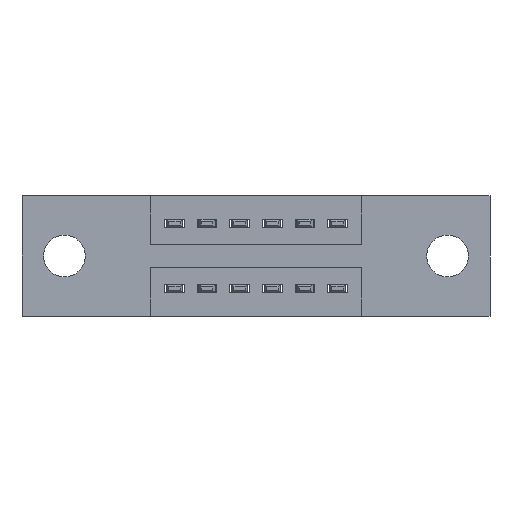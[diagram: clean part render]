
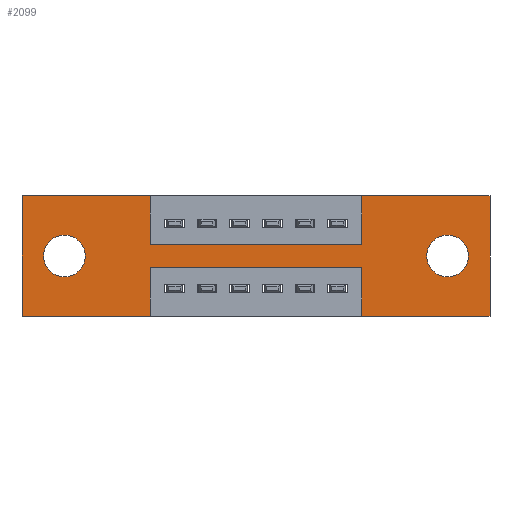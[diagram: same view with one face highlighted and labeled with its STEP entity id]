
A CAD part, front view. The second image highlights one B-rep face of the part: STEP entity #2099.
In plain terms, the highlighted planar face has unit normal (0, -1, 0).
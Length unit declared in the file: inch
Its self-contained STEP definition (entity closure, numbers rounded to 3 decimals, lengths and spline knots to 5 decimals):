
#1 = DIRECTION ( 'NONE',  ( 0., 1., 0. ) ) ;
#26 = CARTESIAN_POINT ( 'NONE',  ( 0., 0., 0. ) ) ;
#52 = EDGE_CURVE ( 'NONE', #2543, #3641, #4441, .T. ) ;
#180 = DIRECTION ( 'NONE',  ( 0., 0., -1. ) ) ;
#314 = VECTOR ( 'NONE', #6771, 39.37008 ) ;
#484 = AXIS2_PLACEMENT_3D ( 'NONE', #5049, #4975, #4965 ) ;
#531 = CARTESIAN_POINT ( 'NONE',  ( 1.305, 0., -0.185 ) ) ;
#575 = DIRECTION ( 'NONE',  ( 0., 0., 1. ) ) ;
#579 = ORIENTED_EDGE ( 'NONE', *, *, #7666, .T. ) ;
#630 = AXIS2_PLACEMENT_3D ( 'NONE', #892, #879, #575 ) ;
#729 = ORIENTED_EDGE ( 'NONE', *, *, #5892, .F. ) ;
#764 = VECTOR ( 'NONE', #1895, 39.37008 ) ;
#770 = LINE ( 'NONE', #5161, #6510 ) ;
#814 = LINE ( 'NONE', #9161, #8529 ) ;
#859 = ORIENTED_EDGE ( 'NONE', *, *, #7295, .F. ) ;
#872 = CARTESIAN_POINT ( 'NONE',  ( 0.3925, 0., -0.37 ) ) ;
#879 = DIRECTION ( 'NONE',  ( 0., 1., 0. ) ) ;
#892 = CARTESIAN_POINT ( 'NONE',  ( 0.13, 0., -0.185 ) ) ;
#940 = VERTEX_POINT ( 'NONE', #3527 ) ;
#981 = VERTEX_POINT ( 'NONE', #2185 ) ;
#990 = ORIENTED_EDGE ( 'NONE', *, *, #2960, .T. ) ;
#1018 = ORIENTED_EDGE ( 'NONE', *, *, #2408, .T. ) ;
#1060 = EDGE_CURVE ( 'NONE', #2987, #3016, #2873, .T. ) ;
#1078 = ORIENTED_EDGE ( 'NONE', *, *, #1060, .F. ) ;
#1226 = ORIENTED_EDGE ( 'NONE', *, *, #8781, .F. ) ;
#1514 = CIRCLE ( 'NONE', #484, 0.064 ) ;
#1549 = ORIENTED_EDGE ( 'NONE', *, *, #4162, .F. ) ;
#1569 = EDGE_LOOP ( 'NONE', ( #990, #1018 ) ) ;
#1657 = ORIENTED_EDGE ( 'NONE', *, *, #9216, .F. ) ;
#1735 = VERTEX_POINT ( 'NONE', #6779 ) ;
#1806 = ORIENTED_EDGE ( 'NONE', *, *, #8166, .F. ) ;
#1809 = DIRECTION ( 'NONE',  ( 0., 0., -1. ) ) ;
#1895 = DIRECTION ( 'NONE',  ( 0., 0., 1. ) ) ;
#1947 = CARTESIAN_POINT ( 'NONE',  ( 1.0425, 0., 0. ) ) ;
#2099 = ADVANCED_FACE ( 'NONE', ( #2370, #7669, #4164 ), #7871, .T. ) ;
#2115 = ORIENTED_EDGE ( 'NONE', *, *, #4120, .F. ) ;
#2185 = CARTESIAN_POINT ( 'NONE',  ( 1.435, 0., -0.37 ) ) ;
#2215 = VERTEX_POINT ( 'NONE', #6495 ) ;
#2240 = CARTESIAN_POINT ( 'NONE',  ( 1.435, 0., 0. ) ) ;
#2258 = ORIENTED_EDGE ( 'NONE', *, *, #8066, .F. ) ;
#2370 = FACE_BOUND ( 'NONE', #1569, .T. ) ;
#2408 = EDGE_CURVE ( 'NONE', #2215, #940, #1514, .T. ) ;
#2412 = ORIENTED_EDGE ( 'NONE', *, *, #52, .F. ) ;
#2415 = CARTESIAN_POINT ( 'NONE',  ( 1.0425, 0., -0.37 ) ) ;
#2441 = EDGE_CURVE ( 'NONE', #3881, #3059, #7356, .T. ) ;
#2543 = VERTEX_POINT ( 'NONE', #3955 ) ;
#2873 = LINE ( 'NONE', #2415, #764 ) ;
#2920 = ORIENTED_EDGE ( 'NONE', *, *, #7743, .F. ) ;
#2931 = CARTESIAN_POINT ( 'NONE',  ( 0., 0., 0. ) ) ;
#2960 = EDGE_CURVE ( 'NONE', #940, #2215, #3087, .T. ) ;
#2987 = VERTEX_POINT ( 'NONE', #7639 ) ;
#3016 = VERTEX_POINT ( 'NONE', #6054 ) ;
#3056 = ORIENTED_EDGE ( 'NONE', *, *, #5454, .T. ) ;
#3059 = VERTEX_POINT ( 'NONE', #4786 ) ;
#3087 = CIRCLE ( 'NONE', #7286, 0.064 ) ;
#3143 = CIRCLE ( 'NONE', #630, 0.064 ) ;
#3177 = ORIENTED_EDGE ( 'NONE', *, *, #2441, .F. ) ;
#3354 = VECTOR ( 'NONE', #7906, 39.37008 ) ;
#3527 = CARTESIAN_POINT ( 'NONE',  ( 1.305, 0., -0.121 ) ) ;
#3598 = CARTESIAN_POINT ( 'NONE',  ( 0.13, 0., -0.185 ) ) ;
#3607 = CARTESIAN_POINT ( 'NONE',  ( 0.3925, 0., -0.15 ) ) ;
#3641 = VERTEX_POINT ( 'NONE', #7553 ) ;
#3727 = EDGE_LOOP ( 'NONE', ( #729, #859, #1078, #1226, #1549, #1657, #1806, #2115, #2258, #2412, #2920, #3177 ) ) ;
#3779 = VERTEX_POINT ( 'NONE', #5271 ) ;
#3881 = VERTEX_POINT ( 'NONE', #872 ) ;
#3955 = CARTESIAN_POINT ( 'NONE',  ( 0., 0., 0. ) ) ;
#4080 = CARTESIAN_POINT ( 'NONE',  ( 0.3925, 0., 0. ) ) ;
#4099 = VERTEX_POINT ( 'NONE', #7479 ) ;
#4120 = EDGE_CURVE ( 'NONE', #8926, #1735, #814, .T. ) ;
#4162 = EDGE_CURVE ( 'NONE', #5011, #981, #8125, .T. ) ;
#4164 = FACE_OUTER_BOUND ( 'NONE', #3727, .T. ) ;
#4248 = LINE ( 'NONE', #6148, #5910 ) ;
#4250 = VERTEX_POINT ( 'NONE', #7046 ) ;
#4353 = DIRECTION ( 'NONE',  ( 0., 0., 1. ) ) ;
#4441 = LINE ( 'NONE', #26, #7911 ) ;
#4540 = EDGE_LOOP ( 'NONE', ( #3056, #579 ) ) ;
#4668 = DIRECTION ( 'NONE',  ( -1., 0., 0. ) ) ;
#4669 = DIRECTION ( 'NONE',  ( 0., 0., -1. ) ) ;
#4786 = CARTESIAN_POINT ( 'NONE',  ( 0., 0., -0.37 ) ) ;
#4965 = DIRECTION ( 'NONE',  ( 0., 0., -1. ) ) ;
#4975 = DIRECTION ( 'NONE',  ( 0., 1., 0. ) ) ;
#4993 = LINE ( 'NONE', #8981, #8342 ) ;
#5011 = VERTEX_POINT ( 'NONE', #2240 ) ;
#5016 = AXIS2_PLACEMENT_3D ( 'NONE', #3598, #8461, #4353 ) ;
#5049 = CARTESIAN_POINT ( 'NONE',  ( 1.305, 0., -0.185 ) ) ;
#5110 = CARTESIAN_POINT ( 'NONE',  ( 0., 0., -0.37 ) ) ;
#5135 = DIRECTION ( 'NONE',  ( -1., 0., 0. ) ) ;
#5161 = CARTESIAN_POINT ( 'NONE',  ( 0.3925, 0., -0.37 ) ) ;
#5271 = CARTESIAN_POINT ( 'NONE',  ( 0.13, 0., -0.121 ) ) ;
#5331 = VECTOR ( 'NONE', #4668, 39.37008 ) ;
#5355 = CARTESIAN_POINT ( 'NONE',  ( 0.3925, 0., -0.22 ) ) ;
#5454 = EDGE_CURVE ( 'NONE', #3779, #4250, #3143, .T. ) ;
#5719 = VECTOR ( 'NONE', #1809, 39.37008 ) ;
#5892 = EDGE_CURVE ( 'NONE', #6343, #3881, #770, .T. ) ;
#5910 = VECTOR ( 'NONE', #8820, 39.37008 ) ;
#6054 = CARTESIAN_POINT ( 'NONE',  ( 1.0425, 0., -0.22 ) ) ;
#6148 = CARTESIAN_POINT ( 'NONE',  ( 0., 0., 0. ) ) ;
#6343 = VERTEX_POINT ( 'NONE', #7694 ) ;
#6348 = DIRECTION ( 'NONE',  ( 0., 0., 1. ) ) ;
#6495 = CARTESIAN_POINT ( 'NONE',  ( 1.305, 0., -0.249 ) ) ;
#6510 = VECTOR ( 'NONE', #4669, 39.37008 ) ;
#6698 = VECTOR ( 'NONE', #6348, 39.37008 ) ;
#6771 = DIRECTION ( 'NONE',  ( 0., 0., -1. ) ) ;
#6779 = CARTESIAN_POINT ( 'NONE',  ( 1.0425, 0., -0.15 ) ) ;
#6795 = CARTESIAN_POINT ( 'NONE',  ( 1.435, 0., 0. ) ) ;
#6850 = DIRECTION ( 'NONE',  ( 1., 0., 0. ) ) ;
#7046 = CARTESIAN_POINT ( 'NONE',  ( 0.13, 0., -0.249 ) ) ;
#7146 = VECTOR ( 'NONE', #5135, 39.37008 ) ;
#7157 = LINE ( 'NONE', #5355, #5331 ) ;
#7286 = AXIS2_PLACEMENT_3D ( 'NONE', #531, #1, #180 ) ;
#7295 = EDGE_CURVE ( 'NONE', #3016, #6343, #7157, .T. ) ;
#7356 = LINE ( 'NONE', #5110, #7146 ) ;
#7479 = CARTESIAN_POINT ( 'NONE',  ( 1.0425, 0., 0. ) ) ;
#7553 = CARTESIAN_POINT ( 'NONE',  ( 0.3925, 0., 0. ) ) ;
#7569 = LINE ( 'NONE', #4080, #5719 ) ;
#7639 = CARTESIAN_POINT ( 'NONE',  ( 1.0425, 0., -0.37 ) ) ;
#7666 = EDGE_CURVE ( 'NONE', #4250, #3779, #9290, .T. ) ;
#7669 = FACE_BOUND ( 'NONE', #4540, .T. ) ;
#7689 = DIRECTION ( 'NONE',  ( -1., 0., 0. ) ) ;
#7694 = CARTESIAN_POINT ( 'NONE',  ( 0.3925, 0., -0.22 ) ) ;
#7743 = EDGE_CURVE ( 'NONE', #3059, #2543, #8683, .T. ) ;
#7790 = DIRECTION ( 'NONE',  ( 0., 0., -1. ) ) ;
#7792 = DIRECTION ( 'NONE',  ( 0., -1., 0. ) ) ;
#7871 = PLANE ( 'NONE',  #9062 ) ;
#7878 = CARTESIAN_POINT ( 'NONE',  ( 0., 0., -0.37 ) ) ;
#7906 = DIRECTION ( 'NONE',  ( 0., 0., 1. ) ) ;
#7911 = VECTOR ( 'NONE', #6850, 39.37008 ) ;
#8066 = EDGE_CURVE ( 'NONE', #3641, #8926, #7569, .T. ) ;
#8125 = LINE ( 'NONE', #6795, #314 ) ;
#8166 = EDGE_CURVE ( 'NONE', #1735, #4099, #8253, .T. ) ;
#8253 = LINE ( 'NONE', #1947, #6698 ) ;
#8342 = VECTOR ( 'NONE', #7689, 39.37008 ) ;
#8461 = DIRECTION ( 'NONE',  ( 0., 1., 0. ) ) ;
#8529 = VECTOR ( 'NONE', #8906, 39.37008 ) ;
#8683 = LINE ( 'NONE', #2931, #3354 ) ;
#8781 = EDGE_CURVE ( 'NONE', #981, #2987, #4993, .T. ) ;
#8820 = DIRECTION ( 'NONE',  ( 1., 0., 0. ) ) ;
#8906 = DIRECTION ( 'NONE',  ( 1., 0., 0. ) ) ;
#8926 = VERTEX_POINT ( 'NONE', #3607 ) ;
#8981 = CARTESIAN_POINT ( 'NONE',  ( 0., 0., -0.37 ) ) ;
#9062 = AXIS2_PLACEMENT_3D ( 'NONE', #7878, #7792, #7790 ) ;
#9161 = CARTESIAN_POINT ( 'NONE',  ( 0.3925, 0., -0.15 ) ) ;
#9216 = EDGE_CURVE ( 'NONE', #4099, #5011, #4248, .T. ) ;
#9290 = CIRCLE ( 'NONE', #5016, 0.064 ) ;
